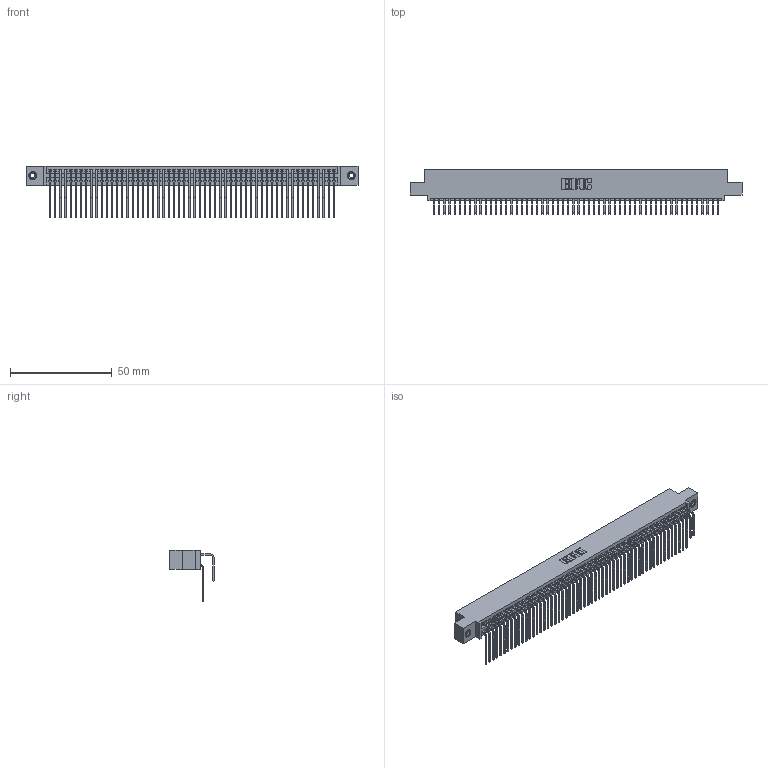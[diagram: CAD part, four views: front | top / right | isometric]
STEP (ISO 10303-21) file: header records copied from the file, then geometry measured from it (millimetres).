
FILE_DESCRIPTION (( 'STEP AP203' ), '1' );
FILE_NAME ('395-112-558-508.STEP', '2018-12-01T12:10:56', ( '' ), ( '' ), 'SwSTEP 2.0', 'SolidWorks 2016', '' );
FILE_SCHEMA (( 'CONFIG_CONTROL_DESIGN' ));
Length unit declared in the file: inch
Products named in the file (5): 395-112-558-508; 345 Part_0.110 Offset - 0.156 Dia-TI; 345-292-001_558 559 Tail - 1; 345-250-001_345-250-003-102; 345-292-001_558 Tail - 2
Assembly tree (115 placements, depth 2):
  395-112-558-508
    345 Part_0.110 Offset - 0.156 Dia-TI
    345-292-001_558 559 Tail - 1  x56
    345-292-001_558 Tail - 2  x56
    345-250-001_345-250-003-102  x2
Bounding box: 163.45 x 21.83 x 25.53 mm (x, y, z)
Volume: 16573.8 mm3; surface area: 27914.4 mm2
Topology: 115 solids, 115 shells, 6014 faces, 17849 edges, 11742 vertices
Faces by surface type: plane 4036, cylinder 1962, cone 12, torus 4
Entity records: 45024 total; most frequent: CARTESIAN_POINT 7562, ORIENTED_EDGE 7438, DIRECTION 6649, EDGE_CURVE 3719, VECTOR 3303, LINE 3303, VERTEX_POINT 2472, AXIS2_PLACEMENT_3D 1673
